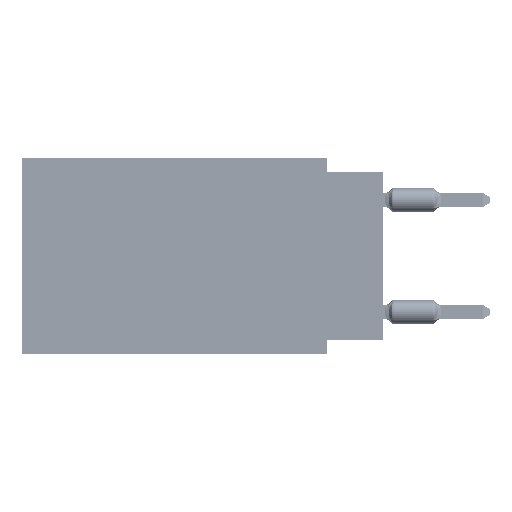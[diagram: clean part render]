
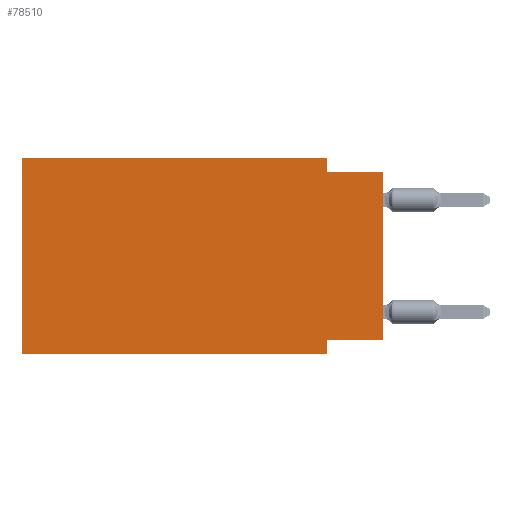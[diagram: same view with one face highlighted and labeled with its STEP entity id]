
A CAD part, left-side view. The second image highlights one B-rep face of the part: STEP entity #78510.
In plain terms, the highlighted planar face has unit normal (-1, 0, 0).
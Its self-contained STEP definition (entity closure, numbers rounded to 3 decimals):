
#239 = VECTOR ( 'NONE', #99100, 1000. ) ;
#1171 = CARTESIAN_POINT ( 'NONE',  ( 0., 0., -8.255 ) ) ;
#3967 = EDGE_CURVE ( 'NONE', #97658, #60488, #29540, .T. ) ;
#4743 = PLANE ( 'NONE',  #42740 ) ;
#5053 = LINE ( 'NONE', #36054, #51343 ) ;
#8700 = VERTEX_POINT ( 'NONE', #82530 ) ;
#9747 = EDGE_CURVE ( 'NONE', #8700, #58547, #5053, .T. ) ;
#10368 = VERTEX_POINT ( 'NONE', #23053 ) ;
#13676 = EDGE_LOOP ( 'NONE', ( #83672, #81673, #34702, #70697, #49560, #65439, #87041, #77649 ) ) ;
#18170 = CARTESIAN_POINT ( 'NONE',  ( 0., 0., -0.635 ) ) ;
#20064 = DIRECTION ( 'NONE',  ( 0., 1., 0. ) ) ;
#20373 = CARTESIAN_POINT ( 'NONE',  ( 0., 16.383, 0. ) ) ;
#21823 = CARTESIAN_POINT ( 'NONE',  ( 0., 0., -0.635 ) ) ;
#23053 = CARTESIAN_POINT ( 'NONE',  ( 0., 16.383, -8.89 ) ) ;
#25587 = EDGE_CURVE ( 'NONE', #97658, #81871, #50017, .T. ) ;
#27208 = CARTESIAN_POINT ( 'NONE',  ( 0., 0., -8.255 ) ) ;
#27458 = DIRECTION ( 'NONE',  ( 0., 0., -1. ) ) ;
#27649 = FACE_OUTER_BOUND ( 'NONE', #13676, .T. ) ;
#28140 = CARTESIAN_POINT ( 'NONE',  ( 0., 16.383, 0. ) ) ;
#29004 = LINE ( 'NONE', #20373, #94779 ) ;
#29037 = EDGE_CURVE ( 'NONE', #10368, #70989, #32157, .T. ) ;
#29540 = LINE ( 'NONE', #52886, #239 ) ;
#29834 = CARTESIAN_POINT ( 'NONE',  ( 0., 2.54, -8.89 ) ) ;
#30982 = EDGE_CURVE ( 'NONE', #81871, #32268, #51683, .T. ) ;
#32157 = LINE ( 'NONE', #55975, #32697 ) ;
#32268 = VERTEX_POINT ( 'NONE', #79850 ) ;
#32697 = VECTOR ( 'NONE', #79351, 1000. ) ;
#34702 = ORIENTED_EDGE ( 'NONE', *, *, #9747, .F. ) ;
#35256 = DIRECTION ( 'NONE',  ( 1., 0., 0. ) ) ;
#36054 = CARTESIAN_POINT ( 'NONE',  ( 0., 2.54, 0. ) ) ;
#36883 = CARTESIAN_POINT ( 'NONE',  ( 0., 2.54, -0.635 ) ) ;
#39126 = DIRECTION ( 'NONE',  ( 0., -1., 0. ) ) ;
#42740 = AXIS2_PLACEMENT_3D ( 'NONE', #28140, #35256, #72333 ) ;
#49560 = ORIENTED_EDGE ( 'NONE', *, *, #29037, .F. ) ;
#50017 = LINE ( 'NONE', #27208, #76028 ) ;
#51343 = VECTOR ( 'NONE', #27458, 1000. ) ;
#51683 = LINE ( 'NONE', #29834, #54067 ) ;
#52886 = CARTESIAN_POINT ( 'NONE',  ( 0., 0., 0. ) ) ;
#54067 = VECTOR ( 'NONE', #76063, 1000. ) ;
#55975 = CARTESIAN_POINT ( 'NONE',  ( 0., 16.383, 0. ) ) ;
#58547 = VERTEX_POINT ( 'NONE', #36883 ) ;
#59929 = LINE ( 'NONE', #21823, #92353 ) ;
#60488 = VERTEX_POINT ( 'NONE', #18170 ) ;
#65439 = ORIENTED_EDGE ( 'NONE', *, *, #70856, .T. ) ;
#68157 = EDGE_CURVE ( 'NONE', #70989, #8700, #29004, .T. ) ;
#70613 = CARTESIAN_POINT ( 'NONE',  ( 0., 16.383, -8.89 ) ) ;
#70697 = ORIENTED_EDGE ( 'NONE', *, *, #68157, .F. ) ;
#70856 = EDGE_CURVE ( 'NONE', #10368, #32268, #93458, .T. ) ;
#70989 = VERTEX_POINT ( 'NONE', #96949 ) ;
#72333 = DIRECTION ( 'NONE',  ( 0., 0., -1. ) ) ;
#76028 = VECTOR ( 'NONE', #20064, 1000. ) ;
#76063 = DIRECTION ( 'NONE',  ( 0., 0., -1. ) ) ;
#76209 = DIRECTION ( 'NONE',  ( 0., -1., 0. ) ) ;
#76659 = CARTESIAN_POINT ( 'NONE',  ( 0., 2.54, -8.255 ) ) ;
#77649 = ORIENTED_EDGE ( 'NONE', *, *, #25587, .F. ) ;
#78510 = ADVANCED_FACE ( 'NONE', ( #27649 ), #4743, .F. ) ;
#79351 = DIRECTION ( 'NONE',  ( 0., 0., 1. ) ) ;
#79850 = CARTESIAN_POINT ( 'NONE',  ( 0., 2.54, -8.89 ) ) ;
#81673 = ORIENTED_EDGE ( 'NONE', *, *, #87539, .F. ) ;
#81871 = VERTEX_POINT ( 'NONE', #76659 ) ;
#82530 = CARTESIAN_POINT ( 'NONE',  ( 0., 2.54, 0. ) ) ;
#83672 = ORIENTED_EDGE ( 'NONE', *, *, #3967, .T. ) ;
#87041 = ORIENTED_EDGE ( 'NONE', *, *, #30982, .F. ) ;
#87539 = EDGE_CURVE ( 'NONE', #58547, #60488, #59929, .T. ) ;
#90882 = DIRECTION ( 'NONE',  ( 0., -1., 0. ) ) ;
#91678 = VECTOR ( 'NONE', #39126, 1000. ) ;
#92353 = VECTOR ( 'NONE', #90882, 1000. ) ;
#93458 = LINE ( 'NONE', #70613, #91678 ) ;
#94779 = VECTOR ( 'NONE', #76209, 1000. ) ;
#96949 = CARTESIAN_POINT ( 'NONE',  ( 0., 16.383, 0. ) ) ;
#97658 = VERTEX_POINT ( 'NONE', #1171 ) ;
#99100 = DIRECTION ( 'NONE',  ( 0., 0., 1. ) ) ;
